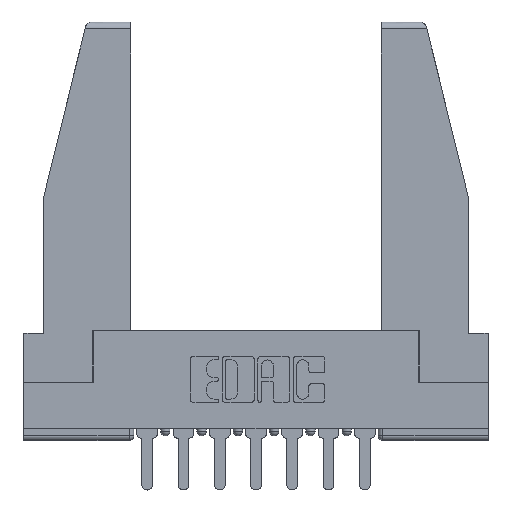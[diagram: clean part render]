
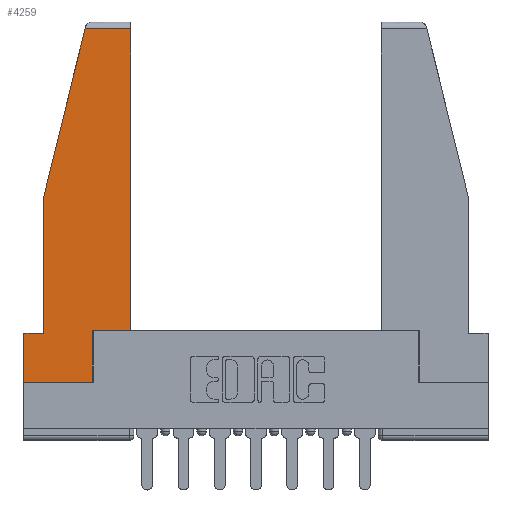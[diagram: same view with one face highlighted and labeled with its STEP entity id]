
A CAD part, top view. The second image highlights one B-rep face of the part: STEP entity #4259.
In plain terms, the highlighted planar face has unit normal (0, 0, 1).
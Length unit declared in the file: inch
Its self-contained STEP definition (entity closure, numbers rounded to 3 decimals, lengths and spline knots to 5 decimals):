
#51 = VERTEX_POINT ( 'NONE', #1824 ) ;
#401 = PLANE ( 'NONE',  #5389 ) ;
#689 = ORIENTED_EDGE ( 'NONE', *, *, #4193, .T. ) ;
#960 = VECTOR ( 'NONE', #9226, 39.37008 ) ;
#1024 = ORIENTED_EDGE ( 'NONE', *, *, #8685, .T. ) ;
#1309 = LINE ( 'NONE', #11439, #11795 ) ;
#1484 = EDGE_CURVE ( 'NONE', #2629, #11428, #12463, .T. ) ;
#1824 = CARTESIAN_POINT ( 'NONE',  ( 0.2636, 1.52, 0. ) ) ;
#1912 = CARTESIAN_POINT ( 'NONE',  ( 0.297, 0., 0. ) ) ;
#1948 = VECTOR ( 'NONE', #12179, 39.37008 ) ;
#2013 = VECTOR ( 'NONE', #7155, 39.37008 ) ;
#2024 = CARTESIAN_POINT ( 'NONE',  ( 0., 0.21, 0. ) ) ;
#2137 = EDGE_CURVE ( 'NONE', #7491, #2629, #7676, .T. ) ;
#2213 = ORIENTED_EDGE ( 'NONE', *, *, #9296, .T. ) ;
#2279 = CARTESIAN_POINT ( 'NONE',  ( 0.271, 1.55, 0. ) ) ;
#2440 = LINE ( 'NONE', #1912, #3552 ) ;
#2472 = EDGE_CURVE ( 'NONE', #4052, #5905, #8424, .T. ) ;
#2559 = DIRECTION ( 'NONE',  ( 0., -1., 0. ) ) ;
#2629 = VERTEX_POINT ( 'NONE', #4651 ) ;
#2698 = VERTEX_POINT ( 'NONE', #3821 ) ;
#2892 = DIRECTION ( 'NONE',  ( 0., 1., 0. ) ) ;
#3165 = VECTOR ( 'NONE', #11695, 39.37008 ) ;
#3342 = EDGE_CURVE ( 'NONE', #11428, #9047, #1309, .T. ) ;
#3406 = DIRECTION ( 'NONE',  ( 0., 0., 1. ) ) ;
#3552 = VECTOR ( 'NONE', #2892, 39.37008 ) ;
#3821 = CARTESIAN_POINT ( 'NONE',  ( 0.086, 0.8, 0. ) ) ;
#4052 = VERTEX_POINT ( 'NONE', #6654 ) ;
#4130 = CARTESIAN_POINT ( 'NONE',  ( 0.297, 0.223, 0. ) ) ;
#4193 = EDGE_CURVE ( 'NONE', #11685, #4052, #9463, .T. ) ;
#4237 = VECTOR ( 'NONE', #5121, 39.37008 ) ;
#4259 = ADVANCED_FACE ( 'NONE', ( #5317 ), #401, .T. ) ;
#4536 = DIRECTION ( 'NONE',  ( 1., 0., 0. ) ) ;
#4651 = CARTESIAN_POINT ( 'NONE',  ( 0., 0.21, 0. ) ) ;
#4682 = LINE ( 'NONE', #6141, #2013 ) ;
#5121 = DIRECTION ( 'NONE',  ( 1., 0., 0. ) ) ;
#5317 = FACE_OUTER_BOUND ( 'NONE', #11554, .T. ) ;
#5326 = CARTESIAN_POINT ( 'NONE',  ( 0.461, 0.223, 0. ) ) ;
#5389 = AXIS2_PLACEMENT_3D ( 'NONE', #12102, #3406, #12182 ) ;
#5722 = CARTESIAN_POINT ( 'NONE',  ( 0.297, 0., 0. ) ) ;
#5905 = VERTEX_POINT ( 'NONE', #8759 ) ;
#6141 = CARTESIAN_POINT ( 'NONE',  ( 0., 1.52, 0. ) ) ;
#6345 = ORIENTED_EDGE ( 'NONE', *, *, #10268, .T. ) ;
#6364 = LINE ( 'NONE', #2279, #960 ) ;
#6654 = CARTESIAN_POINT ( 'NONE',  ( 0.461, 0.223, 0. ) ) ;
#6667 = EDGE_CURVE ( 'NONE', #2698, #7491, #9501, .T. ) ;
#6847 = ORIENTED_EDGE ( 'NONE', *, *, #2137, .T. ) ;
#7155 = DIRECTION ( 'NONE',  ( -1., 0., 0. ) ) ;
#7223 = CARTESIAN_POINT ( 'NONE',  ( 0., 0., 0. ) ) ;
#7491 = VERTEX_POINT ( 'NONE', #10296 ) ;
#7676 = LINE ( 'NONE', #2024, #9821 ) ;
#7785 = CARTESIAN_POINT ( 'NONE',  ( 0.086, 0.8, 0. ) ) ;
#7844 = VECTOR ( 'NONE', #2559, 39.37008 ) ;
#8050 = ORIENTED_EDGE ( 'NONE', *, *, #6667, .T. ) ;
#8424 = LINE ( 'NONE', #5326, #1948 ) ;
#8476 = CARTESIAN_POINT ( 'NONE',  ( 0., 0.21, 0. ) ) ;
#8566 = ORIENTED_EDGE ( 'NONE', *, *, #2472, .T. ) ;
#8685 = EDGE_CURVE ( 'NONE', #51, #2698, #6364, .T. ) ;
#8700 = ORIENTED_EDGE ( 'NONE', *, *, #3342, .T. ) ;
#8759 = CARTESIAN_POINT ( 'NONE',  ( 0.461, 1.52, 0. ) ) ;
#9047 = VERTEX_POINT ( 'NONE', #5722 ) ;
#9226 = DIRECTION ( 'NONE',  ( -0.239, -0.971, 0. ) ) ;
#9296 = EDGE_CURVE ( 'NONE', #5905, #51, #4682, .T. ) ;
#9463 = LINE ( 'NONE', #4130, #4237 ) ;
#9501 = LINE ( 'NONE', #7785, #3165 ) ;
#9821 = VECTOR ( 'NONE', #11890, 39.37008 ) ;
#10268 = EDGE_CURVE ( 'NONE', #9047, #11685, #2440, .T. ) ;
#10296 = CARTESIAN_POINT ( 'NONE',  ( 0.086, 0.21, 0. ) ) ;
#10411 = CARTESIAN_POINT ( 'NONE',  ( 0.297, 0.223, 0. ) ) ;
#11428 = VERTEX_POINT ( 'NONE', #7223 ) ;
#11439 = CARTESIAN_POINT ( 'NONE',  ( 0., 0., 0. ) ) ;
#11554 = EDGE_LOOP ( 'NONE', ( #8566, #2213, #1024, #8050, #6847, #12281, #8700, #6345, #689 ) ) ;
#11685 = VERTEX_POINT ( 'NONE', #10411 ) ;
#11695 = DIRECTION ( 'NONE',  ( 0., -1., 0. ) ) ;
#11795 = VECTOR ( 'NONE', #4536, 39.37008 ) ;
#11890 = DIRECTION ( 'NONE',  ( -1., 0., 0. ) ) ;
#12102 = CARTESIAN_POINT ( 'NONE',  ( 0., 0., 0. ) ) ;
#12179 = DIRECTION ( 'NONE',  ( 0., 1., 0. ) ) ;
#12182 = DIRECTION ( 'NONE',  ( 1., 0., 0. ) ) ;
#12281 = ORIENTED_EDGE ( 'NONE', *, *, #1484, .T. ) ;
#12463 = LINE ( 'NONE', #8476, #7844 ) ;
